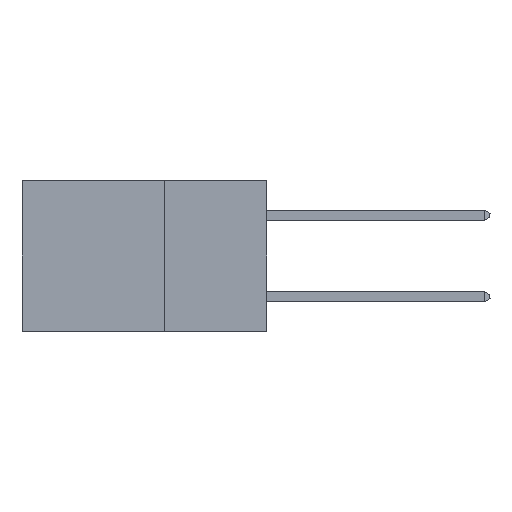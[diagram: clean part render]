
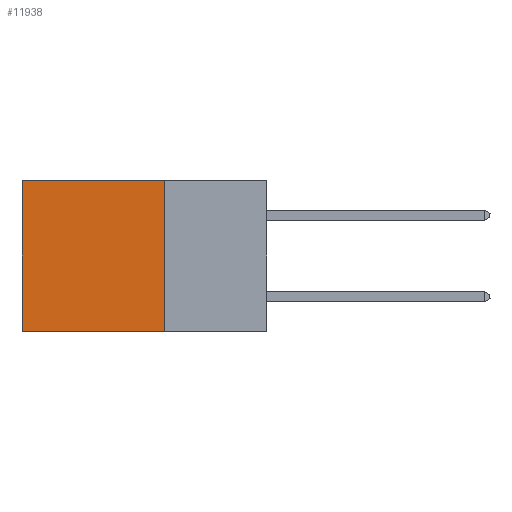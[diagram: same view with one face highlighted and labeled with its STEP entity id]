
A CAD part, left-side view. The second image highlights one B-rep face of the part: STEP entity #11938.
In plain terms, the highlighted planar face has unit normal (-1, 0, 0).
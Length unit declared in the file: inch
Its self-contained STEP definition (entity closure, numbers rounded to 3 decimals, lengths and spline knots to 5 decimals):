
#63 = VERTEX_POINT ( 'NONE', #22912 ) ;
#905 = ORIENTED_EDGE ( 'NONE', *, *, #10178, .F. ) ;
#3422 = FACE_OUTER_BOUND ( 'NONE', #29207, .T. ) ;
#5676 = EDGE_CURVE ( 'NONE', #26210, #10945, #32999, .T. ) ;
#5954 = CARTESIAN_POINT ( 'NONE',  ( 0.2875, 0.6, 0. ) ) ;
#6422 = VECTOR ( 'NONE', #13794, 39.37008 ) ;
#6617 = VERTEX_POINT ( 'NONE', #31801 ) ;
#8858 = CARTESIAN_POINT ( 'NONE',  ( 0.2875, 0.25, -0.37 ) ) ;
#9073 = VECTOR ( 'NONE', #31711, 39.37008 ) ;
#9956 = DIRECTION ( 'NONE',  ( 0., 0., -1. ) ) ;
#10178 = EDGE_CURVE ( 'NONE', #63, #10945, #34619, .T. ) ;
#10945 = VERTEX_POINT ( 'NONE', #16035 ) ;
#11938 = ADVANCED_FACE ( 'NONE', ( #3422 ), #24070, .F. ) ;
#12496 = ORIENTED_EDGE ( 'NONE', *, *, #28881, .F. ) ;
#13794 = DIRECTION ( 'NONE',  ( 0., 0., -1. ) ) ;
#14339 = AXIS2_PLACEMENT_3D ( 'NONE', #20707, #23911, #27167 ) ;
#14375 = ORIENTED_EDGE ( 'NONE', *, *, #5676, .T. ) ;
#16035 = CARTESIAN_POINT ( 'NONE',  ( 0.2875, 0.6, -0.37 ) ) ;
#18060 = VECTOR ( 'NONE', #27393, 39.37008 ) ;
#19181 = CARTESIAN_POINT ( 'NONE',  ( 0.2875, 0.25, 0. ) ) ;
#20707 = CARTESIAN_POINT ( 'NONE',  ( 0.2875, 0.25, 0. ) ) ;
#22912 = CARTESIAN_POINT ( 'NONE',  ( 0.2875, 0.25, -0.37 ) ) ;
#23911 = DIRECTION ( 'NONE',  ( 1., 0., 0. ) ) ;
#24070 = PLANE ( 'NONE',  #14339 ) ;
#25564 = LINE ( 'NONE', #19181, #33097 ) ;
#25902 = EDGE_CURVE ( 'NONE', #6617, #26210, #37602, .T. ) ;
#26210 = VERTEX_POINT ( 'NONE', #5954 ) ;
#26257 = CARTESIAN_POINT ( 'NONE',  ( 0.2875, 0.6, 0. ) ) ;
#27167 = DIRECTION ( 'NONE',  ( 0., 0., -1. ) ) ;
#27393 = DIRECTION ( 'NONE',  ( 0., 1., 0. ) ) ;
#28289 = ORIENTED_EDGE ( 'NONE', *, *, #25902, .T. ) ;
#28881 = EDGE_CURVE ( 'NONE', #6617, #63, #25564, .T. ) ;
#29207 = EDGE_LOOP ( 'NONE', ( #14375, #905, #12496, #28289 ) ) ;
#30506 = CARTESIAN_POINT ( 'NONE',  ( 0.2875, 0.25, 0. ) ) ;
#31711 = DIRECTION ( 'NONE',  ( 0., 1., 0. ) ) ;
#31801 = CARTESIAN_POINT ( 'NONE',  ( 0.2875, 0.25, 0. ) ) ;
#32999 = LINE ( 'NONE', #26257, #6422 ) ;
#33097 = VECTOR ( 'NONE', #9956, 39.37008 ) ;
#34619 = LINE ( 'NONE', #8858, #9073 ) ;
#37602 = LINE ( 'NONE', #30506, #18060 ) ;
